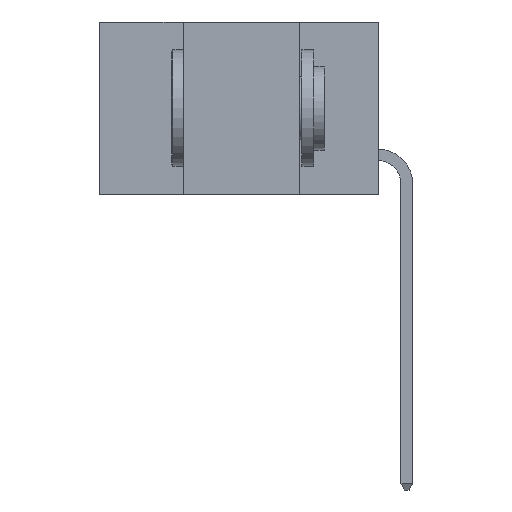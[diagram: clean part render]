
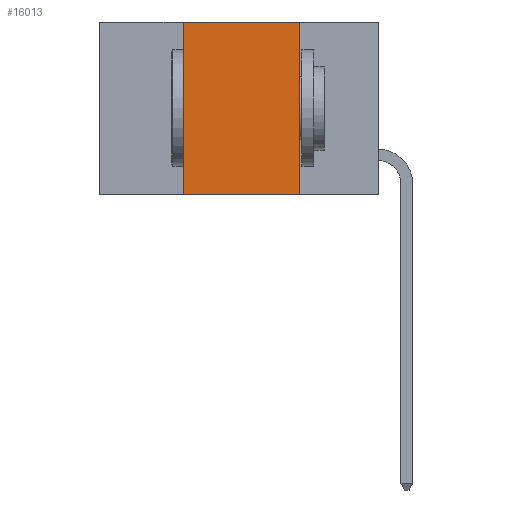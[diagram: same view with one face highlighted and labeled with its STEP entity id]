
A CAD part, left-side view. The second image highlights one B-rep face of the part: STEP entity #16013.
In plain terms, the highlighted planar face has unit normal (-1, 0, 0).
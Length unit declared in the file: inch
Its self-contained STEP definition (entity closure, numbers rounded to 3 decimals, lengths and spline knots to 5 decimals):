
#824 = EDGE_CURVE ( 'NONE', #16684, #3598, #11806, .T. ) ;
#1236 = CARTESIAN_POINT ( 'NONE',  ( 0., 0.6, -0.37 ) ) ;
#1434 = DIRECTION ( 'NONE',  ( 0., 0., 1. ) ) ;
#1517 = CARTESIAN_POINT ( 'NONE',  ( 0., 0.42, -0.37 ) ) ;
#3013 = CARTESIAN_POINT ( 'NONE',  ( 0., 0.6, 0. ) ) ;
#3598 = VERTEX_POINT ( 'NONE', #6116 ) ;
#3714 = VERTEX_POINT ( 'NONE', #4067 ) ;
#4019 = VERTEX_POINT ( 'NONE', #8671 ) ;
#4067 = CARTESIAN_POINT ( 'NONE',  ( 0., 0.17, 0. ) ) ;
#4708 = DIRECTION ( 'NONE',  ( 0., -1., 0. ) ) ;
#4750 = LINE ( 'NONE', #16152, #14820 ) ;
#5111 = DIRECTION ( 'NONE',  ( 0., 0., -1. ) ) ;
#5619 = ORIENTED_EDGE ( 'NONE', *, *, #13312, .F. ) ;
#6116 = CARTESIAN_POINT ( 'NONE',  ( 0., 0.42, 0. ) ) ;
#7070 = VECTOR ( 'NONE', #1434, 39.37008 ) ;
#7187 = ORIENTED_EDGE ( 'NONE', *, *, #824, .F. ) ;
#7565 = ORIENTED_EDGE ( 'NONE', *, *, #19198, .F. ) ;
#8671 = CARTESIAN_POINT ( 'NONE',  ( 0., 0.17, -0.37 ) ) ;
#10427 = EDGE_LOOP ( 'NONE', ( #5619, #7565, #7187, #20393 ) ) ;
#11158 = PLANE ( 'NONE',  #11557 ) ;
#11296 = FACE_OUTER_BOUND ( 'NONE', #10427, .T. ) ;
#11557 = AXIS2_PLACEMENT_3D ( 'NONE', #3013, #17165, #5111 ) ;
#11599 = VECTOR ( 'NONE', #21500, 39.37008 ) ;
#11806 = LINE ( 'NONE', #1517, #7070 ) ;
#12226 = LINE ( 'NONE', #1236, #11599 ) ;
#13312 = EDGE_CURVE ( 'NONE', #3714, #4019, #4750, .T. ) ;
#14737 = CARTESIAN_POINT ( 'NONE',  ( 0., 0.6, 0. ) ) ;
#14820 = VECTOR ( 'NONE', #18204, 39.37008 ) ;
#15751 = VECTOR ( 'NONE', #4708, 39.37008 ) ;
#16013 = ADVANCED_FACE ( 'NONE', ( #11296 ), #11158, .F. ) ;
#16152 = CARTESIAN_POINT ( 'NONE',  ( 0., 0.17, -0.37 ) ) ;
#16387 = LINE ( 'NONE', #14737, #15751 ) ;
#16684 = VERTEX_POINT ( 'NONE', #21200 ) ;
#17165 = DIRECTION ( 'NONE',  ( 1., 0., 0. ) ) ;
#18204 = DIRECTION ( 'NONE',  ( 0., 0., -1. ) ) ;
#19198 = EDGE_CURVE ( 'NONE', #3598, #3714, #16387, .T. ) ;
#20393 = ORIENTED_EDGE ( 'NONE', *, *, #23487, .T. ) ;
#21200 = CARTESIAN_POINT ( 'NONE',  ( 0., 0.42, -0.37 ) ) ;
#21500 = DIRECTION ( 'NONE',  ( 0., -1., 0. ) ) ;
#23487 = EDGE_CURVE ( 'NONE', #16684, #4019, #12226, .T. ) ;
